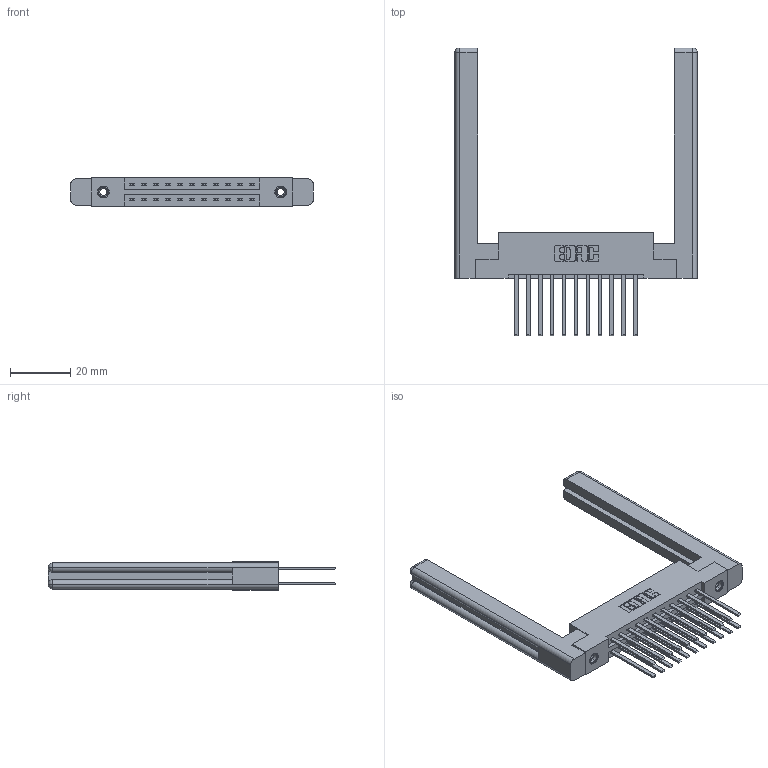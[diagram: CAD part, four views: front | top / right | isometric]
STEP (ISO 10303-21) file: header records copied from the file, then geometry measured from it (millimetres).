
FILE_DESCRIPTION (( 'STEP AP203' ), '1' );
FILE_NAME ('387-022-544-258.STEP', '2019-10-16T17:00:54', ( '' ), ( '' ), 'SwSTEP 2.0', 'SolidWorks 2016', '' );
FILE_SCHEMA (( 'CONFIG_CONTROL_DESIGN' ));
Length unit declared in the file: inch
Products named in the file (5): 307-220-058; 387-022-544-258; 337 Part_Flush Mounting Lugs - 0.156 Dia-TI; 345-250-001_345-250-001-102; 345-292-001_345-293-144
Assembly tree (27 placements, depth 2):
  387-022-544-258
    337 Part_Flush Mounting Lugs - 0.156 Dia-TI
    345-292-001_345-293-144  x22
    345-250-001_345-250-001-102  x2
    307-220-058  x2
Bounding box: 80.21 x 95.38 x 9.4 mm (x, y, z)
Volume: 15491.6 mm3; surface area: 15191.9 mm2
Topology: 27 solids, 27 shells, 1312 faces, 3811 edges, 2498 vertices
Faces by surface type: plane 902, cylinder 386, cone 12, torus 12
Entity records: 14988 total; most frequent: CARTESIAN_POINT 2557, ORIENTED_EDGE 2432, DIRECTION 2244, EDGE_CURVE 1216, VECTOR 1044, LINE 1044, VERTEX_POINT 802, AXIS2_PLACEMENT_3D 600
